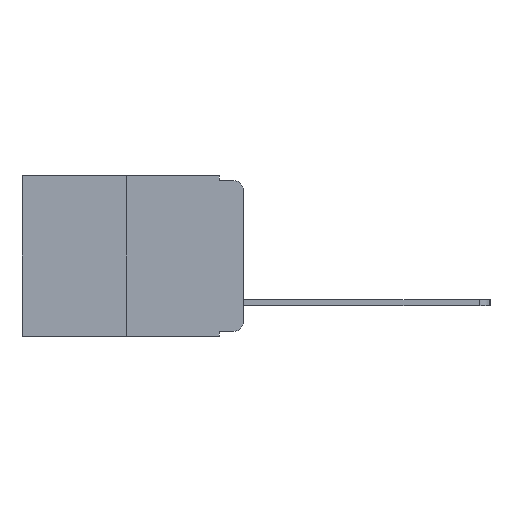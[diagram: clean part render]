
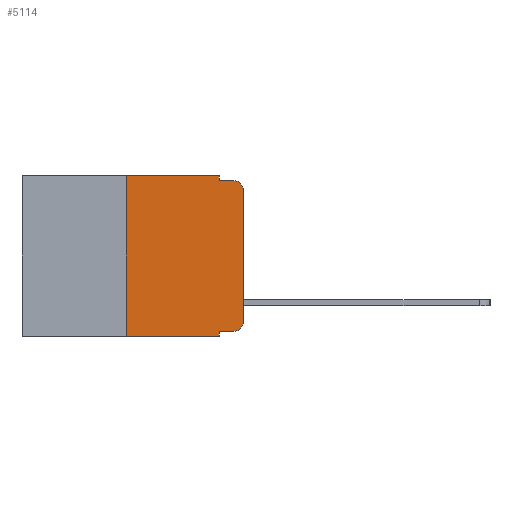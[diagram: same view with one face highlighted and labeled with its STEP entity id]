
A CAD part, left-side view. The second image highlights one B-rep face of the part: STEP entity #5114.
In plain terms, the highlighted planar face has unit normal (-1, 0, 0).
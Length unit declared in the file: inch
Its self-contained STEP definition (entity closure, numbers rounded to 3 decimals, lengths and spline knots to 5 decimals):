
#107 = EDGE_CURVE ( 'NONE', #383, #838, #13909, .T. ) ;
#383 = VERTEX_POINT ( 'NONE', #13337 ) ;
#493 = DIRECTION ( 'NONE',  ( 0., 0., 1. ) ) ;
#552 = EDGE_CURVE ( 'NONE', #11039, #10614, #10203, .T. ) ;
#710 = ORIENTED_EDGE ( 'NONE', *, *, #10394, .T. ) ;
#838 = VERTEX_POINT ( 'NONE', #8862 ) ;
#1135 = VECTOR ( 'NONE', #10755, 39.37008 ) ;
#1218 = CARTESIAN_POINT ( 'NONE',  ( 0., 0.051, 0. ) ) ;
#1443 = ORIENTED_EDGE ( 'NONE', *, *, #552, .F. ) ;
#2576 = CARTESIAN_POINT ( 'NONE',  ( 0., 0., 0. ) ) ;
#2761 = VERTEX_POINT ( 'NONE', #14179 ) ;
#2851 = DIRECTION ( 'NONE',  ( 0., 0., -1. ) ) ;
#3198 = LINE ( 'NONE', #6565, #16049 ) ;
#3333 = DIRECTION ( 'NONE',  ( 0., 0., -1. ) ) ;
#3348 = CARTESIAN_POINT ( 'NONE',  ( 0., 0.473, -0.343 ) ) ;
#3423 = DIRECTION ( 'NONE',  ( 0., 0., -1. ) ) ;
#4321 = VERTEX_POINT ( 'NONE', #19093 ) ;
#4528 = ORIENTED_EDGE ( 'NONE', *, *, #8459, .F. ) ;
#4612 = CARTESIAN_POINT ( 'NONE',  ( 0., 0.02, -0.01 ) ) ;
#4948 = CARTESIAN_POINT ( 'NONE',  ( 0., 0.051, 0. ) ) ;
#5114 = ADVANCED_FACE ( 'NONE', ( #12245 ), #15199, .F. ) ;
#5225 = LINE ( 'NONE', #3348, #16961 ) ;
#5384 = LINE ( 'NONE', #16879, #17612 ) ;
#5527 = LINE ( 'NONE', #8301, #1135 ) ;
#5707 = VERTEX_POINT ( 'NONE', #15263 ) ;
#6274 = DIRECTION ( 'NONE',  ( 0., 0., 1. ) ) ;
#6317 = EDGE_CURVE ( 'NONE', #10614, #17026, #5384, .T. ) ;
#6565 = CARTESIAN_POINT ( 'NONE',  ( 0., 0.051, -0.333 ) ) ;
#6579 = DIRECTION ( 'NONE',  ( -1., 0., 0. ) ) ;
#6669 = DIRECTION ( 'NONE',  ( 0., -1., 0. ) ) ;
#6720 = CARTESIAN_POINT ( 'NONE',  ( 0., 0.25, -0.343 ) ) ;
#6876 = ORIENTED_EDGE ( 'NONE', *, *, #14629, .T. ) ;
#7113 = ORIENTED_EDGE ( 'NONE', *, *, #6317, .F. ) ;
#8078 = EDGE_CURVE ( 'NONE', #17026, #15381, #12594, .T. ) ;
#8301 = CARTESIAN_POINT ( 'NONE',  ( 0., 0.051, -0.01 ) ) ;
#8459 = EDGE_CURVE ( 'NONE', #15381, #11496, #5527, .T. ) ;
#8757 = EDGE_CURVE ( 'NONE', #4321, #383, #18495, .T. ) ;
#8798 = DIRECTION ( 'NONE',  ( 1., 0., 0. ) ) ;
#8807 = CARTESIAN_POINT ( 'NONE',  ( 0., 0.25, 0. ) ) ;
#8862 = CARTESIAN_POINT ( 'NONE',  ( 0., 0., -0.03 ) ) ;
#9046 = CARTESIAN_POINT ( 'NONE',  ( 0., 0.051, 0. ) ) ;
#9115 = DIRECTION ( 'NONE',  ( -1., 0., 0. ) ) ;
#9248 = AXIS2_PLACEMENT_3D ( 'NONE', #18602, #9115, #20151 ) ;
#9686 = VECTOR ( 'NONE', #493, 39.37008 ) ;
#9710 = VECTOR ( 'NONE', #6274, 39.37008 ) ;
#9929 = EDGE_LOOP ( 'NONE', ( #18038, #16326, #4528, #15124, #7113, #1443, #710, #12416, #6876, #9942 ) ) ;
#9942 = ORIENTED_EDGE ( 'NONE', *, *, #8757, .T. ) ;
#10167 = CARTESIAN_POINT ( 'NONE',  ( 0., 0.02, -0.313 ) ) ;
#10203 = LINE ( 'NONE', #15014, #9686 ) ;
#10394 = EDGE_CURVE ( 'NONE', #11039, #2761, #5225, .T. ) ;
#10614 = VERTEX_POINT ( 'NONE', #8807 ) ;
#10755 = DIRECTION ( 'NONE',  ( 0., -1., 0. ) ) ;
#11039 = VERTEX_POINT ( 'NONE', #6720 ) ;
#11496 = VERTEX_POINT ( 'NONE', #4612 ) ;
#12105 = CIRCLE ( 'NONE', #9248, 0.02 ) ;
#12245 = FACE_OUTER_BOUND ( 'NONE', #9929, .T. ) ;
#12416 = ORIENTED_EDGE ( 'NONE', *, *, #14014, .F. ) ;
#12594 = LINE ( 'NONE', #1218, #16292 ) ;
#13337 = CARTESIAN_POINT ( 'NONE',  ( 0., 0., -0.313 ) ) ;
#13816 = CARTESIAN_POINT ( 'NONE',  ( 0., 0.473, 0. ) ) ;
#13909 = LINE ( 'NONE', #2576, #9710 ) ;
#14014 = EDGE_CURVE ( 'NONE', #5707, #2761, #20011, .T. ) ;
#14179 = CARTESIAN_POINT ( 'NONE',  ( 0., 0.051, -0.343 ) ) ;
#14629 = EDGE_CURVE ( 'NONE', #5707, #4321, #3198, .T. ) ;
#15014 = CARTESIAN_POINT ( 'NONE',  ( 0., 0.25, 0. ) ) ;
#15124 = ORIENTED_EDGE ( 'NONE', *, *, #8078, .F. ) ;
#15199 = PLANE ( 'NONE',  #20683 ) ;
#15263 = CARTESIAN_POINT ( 'NONE',  ( 0., 0.051, -0.333 ) ) ;
#15290 = EDGE_CURVE ( 'NONE', #838, #11496, #12105, .T. ) ;
#15354 = VECTOR ( 'NONE', #3333, 39.37008 ) ;
#15381 = VERTEX_POINT ( 'NONE', #15631 ) ;
#15631 = CARTESIAN_POINT ( 'NONE',  ( 0., 0.051, -0.01 ) ) ;
#16049 = VECTOR ( 'NONE', #19304, 39.37008 ) ;
#16292 = VECTOR ( 'NONE', #2851, 39.37008 ) ;
#16326 = ORIENTED_EDGE ( 'NONE', *, *, #15290, .T. ) ;
#16879 = CARTESIAN_POINT ( 'NONE',  ( 0., 0.473, 0. ) ) ;
#16961 = VECTOR ( 'NONE', #6669, 39.37008 ) ;
#17026 = VERTEX_POINT ( 'NONE', #9046 ) ;
#17117 = DIRECTION ( 'NONE',  ( 0., -1., 0. ) ) ;
#17612 = VECTOR ( 'NONE', #17117, 39.37008 ) ;
#17723 = DIRECTION ( 'NONE',  ( 0., 0., -1. ) ) ;
#18038 = ORIENTED_EDGE ( 'NONE', *, *, #107, .T. ) ;
#18495 = CIRCLE ( 'NONE', #20112, 0.02 ) ;
#18602 = CARTESIAN_POINT ( 'NONE',  ( 0., 0.02, -0.03 ) ) ;
#19093 = CARTESIAN_POINT ( 'NONE',  ( 0., 0.02, -0.333 ) ) ;
#19304 = DIRECTION ( 'NONE',  ( 0., -1., 0. ) ) ;
#20011 = LINE ( 'NONE', #4948, #15354 ) ;
#20112 = AXIS2_PLACEMENT_3D ( 'NONE', #10167, #6579, #17723 ) ;
#20151 = DIRECTION ( 'NONE',  ( 0., 0., -1. ) ) ;
#20683 = AXIS2_PLACEMENT_3D ( 'NONE', #13816, #8798, #3423 ) ;
